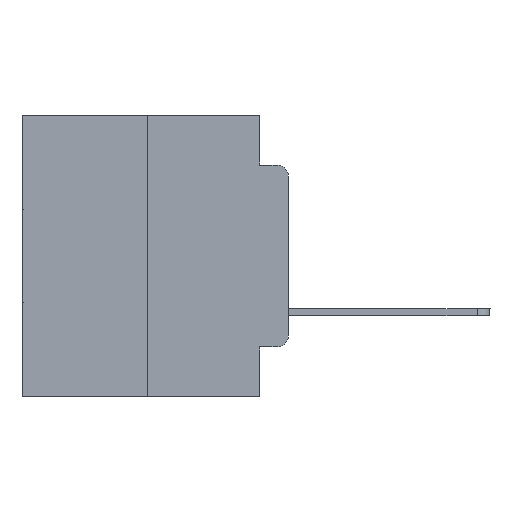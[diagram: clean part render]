
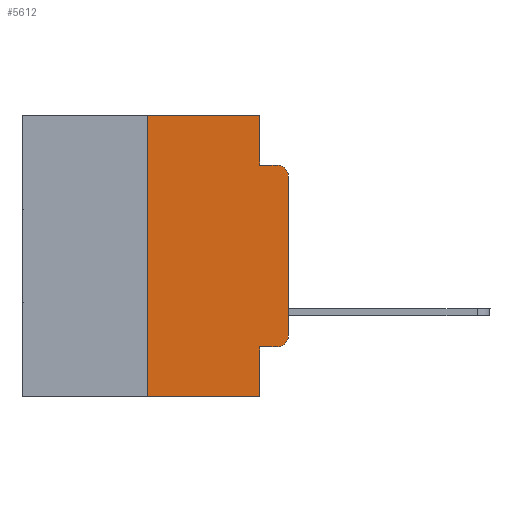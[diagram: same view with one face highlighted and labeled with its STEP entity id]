
A CAD part, left-side view. The second image highlights one B-rep face of the part: STEP entity #5612.
In plain terms, the highlighted planar face has unit normal (-1, 0, 0).
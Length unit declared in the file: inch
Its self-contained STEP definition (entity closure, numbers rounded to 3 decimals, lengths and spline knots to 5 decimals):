
#201 = LINE ( 'NONE', #27835, #21367 ) ;
#569 = EDGE_CURVE ( 'NONE', #9640, #22701, #1122, .T. ) ;
#1001 = DIRECTION ( 'NONE',  ( 0., 0., -1. ) ) ;
#1122 = LINE ( 'NONE', #15032, #3166 ) ;
#1794 = EDGE_LOOP ( 'NONE', ( #3394, #27195, #21558, #21629, #13982, #19817, #21327, #8947, #26890, #9262 ) ) ;
#1801 = VECTOR ( 'NONE', #5695, 39.37008 ) ;
#3036 = CARTESIAN_POINT ( 'NONE',  ( 0., 0., 0. ) ) ;
#3166 = VECTOR ( 'NONE', #7944, 39.37008 ) ;
#3394 = ORIENTED_EDGE ( 'NONE', *, *, #18757, .T. ) ;
#3738 = DIRECTION ( 'NONE',  ( 1., 0., 0. ) ) ;
#4230 = AXIS2_PLACEMENT_3D ( 'NONE', #14922, #28922, #1001 ) ;
#4495 = DIRECTION ( 'NONE',  ( 0., 0., -1. ) ) ;
#4541 = VECTOR ( 'NONE', #21448, 39.37008 ) ;
#5217 = EDGE_CURVE ( 'NONE', #10549, #24042, #29024, .T. ) ;
#5571 = VECTOR ( 'NONE', #6953, 39.37008 ) ;
#5612 = ADVANCED_FACE ( 'NONE', ( #24411 ), #19874, .F. ) ;
#5695 = DIRECTION ( 'NONE',  ( 0., 0., 1. ) ) ;
#5751 = EDGE_CURVE ( 'NONE', #17765, #29217, #201, .T. ) ;
#6588 = EDGE_CURVE ( 'NONE', #21016, #10549, #18396, .T. ) ;
#6907 = LINE ( 'NONE', #25305, #28747 ) ;
#6953 = DIRECTION ( 'NONE',  ( 0., -1., 0. ) ) ;
#7072 = EDGE_CURVE ( 'NONE', #21016, #22701, #25317, .T. ) ;
#7944 = DIRECTION ( 'NONE',  ( 0., -1., 0. ) ) ;
#8947 = ORIENTED_EDGE ( 'NONE', *, *, #7072, .F. ) ;
#9022 = DIRECTION ( 'NONE',  ( 0., -1., 0. ) ) ;
#9262 = ORIENTED_EDGE ( 'NONE', *, *, #5217, .T. ) ;
#9640 = VERTEX_POINT ( 'NONE', #12443 ) ;
#10381 = DIRECTION ( 'NONE',  ( 0., 0., -1. ) ) ;
#10549 = VERTEX_POINT ( 'NONE', #21230 ) ;
#11273 = CARTESIAN_POINT ( 'NONE',  ( 0., 0.051, 0. ) ) ;
#11337 = VERTEX_POINT ( 'NONE', #25843 ) ;
#12443 = CARTESIAN_POINT ( 'NONE',  ( 0., 0.25, -0.5 ) ) ;
#13065 = VERTEX_POINT ( 'NONE', #24722 ) ;
#13982 = ORIENTED_EDGE ( 'NONE', *, *, #5751, .F. ) ;
#14231 = LINE ( 'NONE', #3036, #4541 ) ;
#14922 = CARTESIAN_POINT ( 'NONE',  ( 0., 0.02, -0.1085 ) ) ;
#15032 = CARTESIAN_POINT ( 'NONE',  ( 0., 0.473, -0.5 ) ) ;
#15819 = LINE ( 'NONE', #22761, #18032 ) ;
#15945 = CARTESIAN_POINT ( 'NONE',  ( 0., 0.051, -0.5 ) ) ;
#15994 = CARTESIAN_POINT ( 'NONE',  ( 0., 0.051, -0.4115 ) ) ;
#16971 = AXIS2_PLACEMENT_3D ( 'NONE', #25052, #29264, #29712 ) ;
#17309 = CARTESIAN_POINT ( 'NONE',  ( 0., 0.25, 0. ) ) ;
#17765 = VERTEX_POINT ( 'NONE', #18845 ) ;
#18032 = VECTOR ( 'NONE', #20491, 39.37008 ) ;
#18396 = LINE ( 'NONE', #15994, #5571 ) ;
#18682 = VERTEX_POINT ( 'NONE', #26134 ) ;
#18757 = EDGE_CURVE ( 'NONE', #24042, #18682, #14231, .T. ) ;
#18845 = CARTESIAN_POINT ( 'NONE',  ( 0., 0.25, 0. ) ) ;
#19423 = CARTESIAN_POINT ( 'NONE',  ( 0., 0.051, -0.4115 ) ) ;
#19476 = EDGE_CURVE ( 'NONE', #29217, #11337, #15819, .T. ) ;
#19817 = ORIENTED_EDGE ( 'NONE', *, *, #23890, .F. ) ;
#19874 = PLANE ( 'NONE',  #26154 ) ;
#20491 = DIRECTION ( 'NONE',  ( 0., 0., -1. ) ) ;
#20635 = CARTESIAN_POINT ( 'NONE',  ( 0., 0.051, 0. ) ) ;
#21016 = VERTEX_POINT ( 'NONE', #19423 ) ;
#21230 = CARTESIAN_POINT ( 'NONE',  ( 0., 0.02, -0.4115 ) ) ;
#21327 = ORIENTED_EDGE ( 'NONE', *, *, #569, .T. ) ;
#21367 = VECTOR ( 'NONE', #22714, 39.37008 ) ;
#21448 = DIRECTION ( 'NONE',  ( 0., 0., 1. ) ) ;
#21558 = ORIENTED_EDGE ( 'NONE', *, *, #22807, .F. ) ;
#21566 = CIRCLE ( 'NONE', #4230, 0.02 ) ;
#21629 = ORIENTED_EDGE ( 'NONE', *, *, #19476, .F. ) ;
#22398 = VECTOR ( 'NONE', #4495, 39.37008 ) ;
#22701 = VERTEX_POINT ( 'NONE', #15945 ) ;
#22714 = DIRECTION ( 'NONE',  ( 0., -1., 0. ) ) ;
#22761 = CARTESIAN_POINT ( 'NONE',  ( 0., 0.051, 0. ) ) ;
#22807 = EDGE_CURVE ( 'NONE', #11337, #13065, #6907, .T. ) ;
#23854 = EDGE_CURVE ( 'NONE', #18682, #13065, #21566, .T. ) ;
#23890 = EDGE_CURVE ( 'NONE', #9640, #17765, #24112, .T. ) ;
#23973 = CARTESIAN_POINT ( 'NONE',  ( 0., 0.473, 0. ) ) ;
#24042 = VERTEX_POINT ( 'NONE', #29516 ) ;
#24112 = LINE ( 'NONE', #17309, #1801 ) ;
#24411 = FACE_OUTER_BOUND ( 'NONE', #1794, .T. ) ;
#24722 = CARTESIAN_POINT ( 'NONE',  ( 0., 0.02, -0.0885 ) ) ;
#25052 = CARTESIAN_POINT ( 'NONE',  ( 0., 0.02, -0.3915 ) ) ;
#25305 = CARTESIAN_POINT ( 'NONE',  ( 0., 0.051, -0.0885 ) ) ;
#25317 = LINE ( 'NONE', #20635, #22398 ) ;
#25843 = CARTESIAN_POINT ( 'NONE',  ( 0., 0.051, -0.0885 ) ) ;
#26134 = CARTESIAN_POINT ( 'NONE',  ( 0., 0., -0.1085 ) ) ;
#26154 = AXIS2_PLACEMENT_3D ( 'NONE', #23973, #3738, #10381 ) ;
#26890 = ORIENTED_EDGE ( 'NONE', *, *, #6588, .T. ) ;
#27195 = ORIENTED_EDGE ( 'NONE', *, *, #23854, .T. ) ;
#27835 = CARTESIAN_POINT ( 'NONE',  ( 0., 0.473, 0. ) ) ;
#28747 = VECTOR ( 'NONE', #9022, 39.37008 ) ;
#28922 = DIRECTION ( 'NONE',  ( -1., 0., 0. ) ) ;
#29024 = CIRCLE ( 'NONE', #16971, 0.02 ) ;
#29217 = VERTEX_POINT ( 'NONE', #11273 ) ;
#29264 = DIRECTION ( 'NONE',  ( -1., 0., 0. ) ) ;
#29516 = CARTESIAN_POINT ( 'NONE',  ( 0., 0., -0.3915 ) ) ;
#29712 = DIRECTION ( 'NONE',  ( 0., 0., -1. ) ) ;
